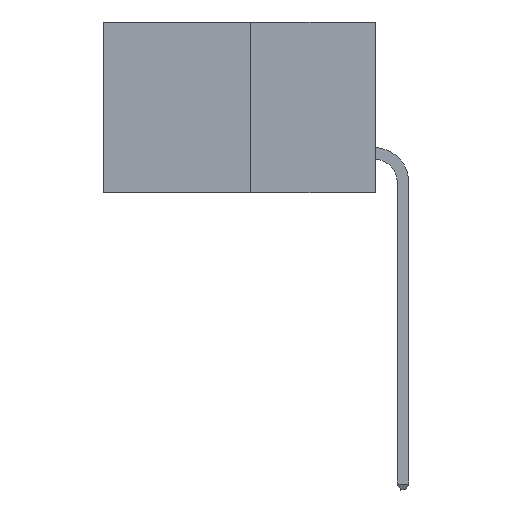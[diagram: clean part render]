
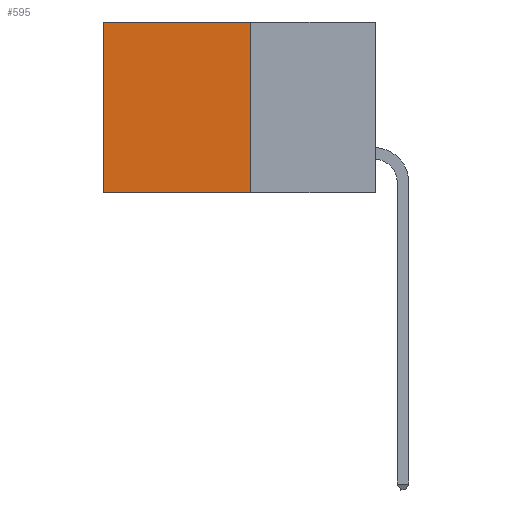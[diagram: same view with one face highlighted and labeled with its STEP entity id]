
A CAD part, left-side view. The second image highlights one B-rep face of the part: STEP entity #595.
In plain terms, the highlighted planar face has unit normal (-1, 0, 0).
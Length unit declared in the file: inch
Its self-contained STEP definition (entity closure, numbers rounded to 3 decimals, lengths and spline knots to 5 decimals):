
#25 = LINE ( 'NONE', #3126, #5116 ) ;
#595 = ADVANCED_FACE ( 'NONE', ( #1359 ), #11452, .F. ) ;
#1359 = FACE_OUTER_BOUND ( 'NONE', #7230, .T. ) ;
#1396 = LINE ( 'NONE', #2358, #3776 ) ;
#1614 = EDGE_CURVE ( 'NONE', #7020, #4306, #11226, .T. ) ;
#1760 = DIRECTION ( 'NONE',  ( 1., 0., 0. ) ) ;
#2358 = CARTESIAN_POINT ( 'NONE',  ( 0.277, 0.27, -0.37 ) ) ;
#2403 = DIRECTION ( 'NONE',  ( 0., 0., -1. ) ) ;
#2993 = CARTESIAN_POINT ( 'NONE',  ( 0.277, 0.59, -0.37 ) ) ;
#3035 = DIRECTION ( 'NONE',  ( 0., 0., -1. ) ) ;
#3041 = VECTOR ( 'NONE', #2403, 39.37008 ) ;
#3097 = EDGE_CURVE ( 'NONE', #8468, #12454, #12088, .T. ) ;
#3126 = CARTESIAN_POINT ( 'NONE',  ( 0.277, 0.27, 0. ) ) ;
#3166 = DIRECTION ( 'NONE',  ( 0., 1., 0. ) ) ;
#3389 = DIRECTION ( 'NONE',  ( 0., 1., 0. ) ) ;
#3506 = CARTESIAN_POINT ( 'NONE',  ( 0.277, 0.27, -0.37 ) ) ;
#3542 = CARTESIAN_POINT ( 'NONE',  ( 0.277, 0.59, 0. ) ) ;
#3728 = EDGE_CURVE ( 'NONE', #7020, #8468, #25, .T. ) ;
#3776 = VECTOR ( 'NONE', #3389, 39.37008 ) ;
#4238 = CARTESIAN_POINT ( 'NONE',  ( 0.277, 0.27, -0.37 ) ) ;
#4306 = VERTEX_POINT ( 'NONE', #4238 ) ;
#4599 = ORIENTED_EDGE ( 'NONE', *, *, #1614, .F. ) ;
#5116 = VECTOR ( 'NONE', #3166, 39.37008 ) ;
#6064 = DIRECTION ( 'NONE',  ( 0., 0., -1. ) ) ;
#6196 = CARTESIAN_POINT ( 'NONE',  ( 0.277, 0.59, -0.37 ) ) ;
#6724 = ORIENTED_EDGE ( 'NONE', *, *, #10427, .F. ) ;
#7020 = VERTEX_POINT ( 'NONE', #10961 ) ;
#7230 = EDGE_LOOP ( 'NONE', ( #11013, #6724, #4599, #10619 ) ) ;
#7345 = VECTOR ( 'NONE', #3035, 39.37008 ) ;
#8022 = CARTESIAN_POINT ( 'NONE',  ( 0.277, 0.27, -0.37 ) ) ;
#8468 = VERTEX_POINT ( 'NONE', #3542 ) ;
#9952 = AXIS2_PLACEMENT_3D ( 'NONE', #8022, #1760, #6064 ) ;
#10427 = EDGE_CURVE ( 'NONE', #4306, #12454, #1396, .T. ) ;
#10619 = ORIENTED_EDGE ( 'NONE', *, *, #3728, .T. ) ;
#10961 = CARTESIAN_POINT ( 'NONE',  ( 0.277, 0.27, 0. ) ) ;
#11013 = ORIENTED_EDGE ( 'NONE', *, *, #3097, .T. ) ;
#11226 = LINE ( 'NONE', #3506, #3041 ) ;
#11452 = PLANE ( 'NONE',  #9952 ) ;
#12088 = LINE ( 'NONE', #2993, #7345 ) ;
#12454 = VERTEX_POINT ( 'NONE', #6196 ) ;
